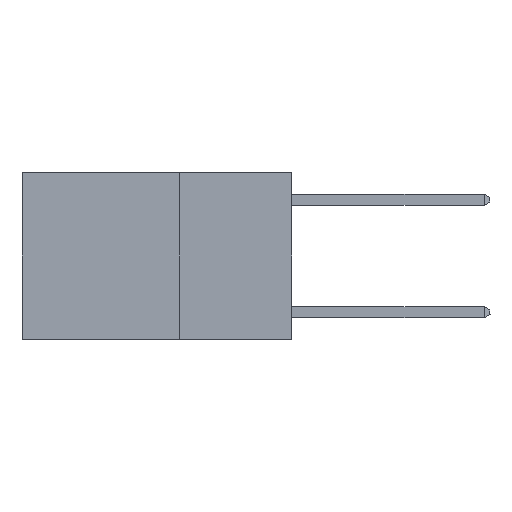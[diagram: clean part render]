
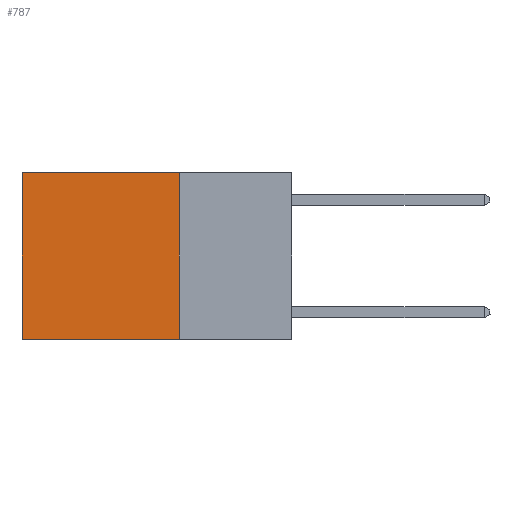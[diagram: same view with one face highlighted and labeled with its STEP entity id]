
A CAD part, left-side view. The second image highlights one B-rep face of the part: STEP entity #787.
In plain terms, the highlighted planar face has unit normal (-1, 0, 0).
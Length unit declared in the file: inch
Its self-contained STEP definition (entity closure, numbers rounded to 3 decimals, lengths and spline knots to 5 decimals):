
#390 = CARTESIAN_POINT ( 'NONE',  ( 0.2625, 0.25, 0. ) ) ;
#445 = ORIENTED_EDGE ( 'NONE', *, *, #721, .T. ) ;
#541 = CARTESIAN_POINT ( 'NONE',  ( 0.2625, 0.6, -0.37 ) ) ;
#721 = EDGE_CURVE ( 'NONE', #11233, #984, #2749, .T. ) ;
#787 = ADVANCED_FACE ( 'NONE', ( #1022 ), #9380, .F. ) ;
#984 = VERTEX_POINT ( 'NONE', #5432 ) ;
#1022 = FACE_OUTER_BOUND ( 'NONE', #7036, .T. ) ;
#1045 = ORIENTED_EDGE ( 'NONE', *, *, #6442, .F. ) ;
#2348 = DIRECTION ( 'NONE',  ( 0., 0., -1. ) ) ;
#2382 = VECTOR ( 'NONE', #5058, 39.37008 ) ;
#2440 = ORIENTED_EDGE ( 'NONE', *, *, #8915, .F. ) ;
#2545 = CARTESIAN_POINT ( 'NONE',  ( 0.2625, 0.6, 0. ) ) ;
#2588 = CARTESIAN_POINT ( 'NONE',  ( 0.2625, 0.25, -0.37 ) ) ;
#2749 = LINE ( 'NONE', #390, #11351 ) ;
#3621 = VECTOR ( 'NONE', #7919, 39.37008 ) ;
#3738 = DIRECTION ( 'NONE',  ( 0., 1., 0. ) ) ;
#3972 = VERTEX_POINT ( 'NONE', #2588 ) ;
#4837 = LINE ( 'NONE', #11176, #2382 ) ;
#5058 = DIRECTION ( 'NONE',  ( 0., 1., 0. ) ) ;
#5432 = CARTESIAN_POINT ( 'NONE',  ( 0.2625, 0.6, 0. ) ) ;
#5496 = LINE ( 'NONE', #2545, #9900 ) ;
#6066 = DIRECTION ( 'NONE',  ( 1., 0., 0. ) ) ;
#6358 = LINE ( 'NONE', #10444, #3621 ) ;
#6442 = EDGE_CURVE ( 'NONE', #11233, #3972, #6358, .T. ) ;
#7036 = EDGE_LOOP ( 'NONE', ( #9486, #2440, #1045, #445 ) ) ;
#7919 = DIRECTION ( 'NONE',  ( 0., 0., -1. ) ) ;
#8363 = AXIS2_PLACEMENT_3D ( 'NONE', #10862, #6066, #2348 ) ;
#8896 = DIRECTION ( 'NONE',  ( 0., 0., -1. ) ) ;
#8915 = EDGE_CURVE ( 'NONE', #3972, #10369, #4837, .T. ) ;
#9380 = PLANE ( 'NONE',  #8363 ) ;
#9486 = ORIENTED_EDGE ( 'NONE', *, *, #11148, .T. ) ;
#9797 = CARTESIAN_POINT ( 'NONE',  ( 0.2625, 0.25, 0. ) ) ;
#9900 = VECTOR ( 'NONE', #8896, 39.37008 ) ;
#10369 = VERTEX_POINT ( 'NONE', #541 ) ;
#10444 = CARTESIAN_POINT ( 'NONE',  ( 0.2625, 0.25, 0. ) ) ;
#10862 = CARTESIAN_POINT ( 'NONE',  ( 0.2625, 0.25, 0. ) ) ;
#11148 = EDGE_CURVE ( 'NONE', #984, #10369, #5496, .T. ) ;
#11176 = CARTESIAN_POINT ( 'NONE',  ( 0.2625, 0.25, -0.37 ) ) ;
#11233 = VERTEX_POINT ( 'NONE', #9797 ) ;
#11351 = VECTOR ( 'NONE', #3738, 39.37008 ) ;
